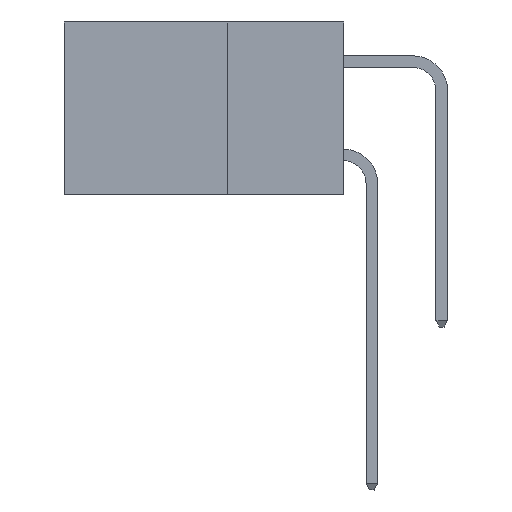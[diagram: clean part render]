
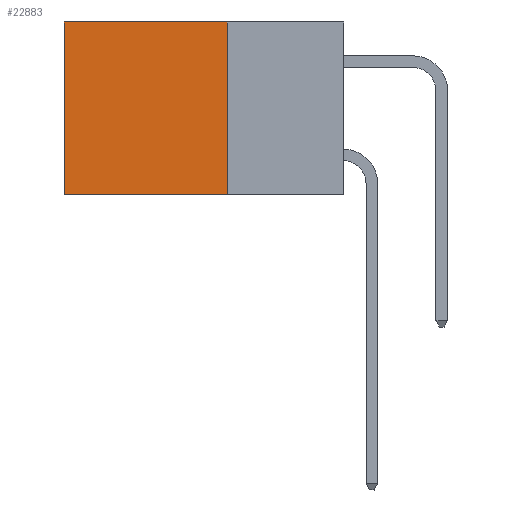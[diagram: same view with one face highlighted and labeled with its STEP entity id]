
A CAD part, left-side view. The second image highlights one B-rep face of the part: STEP entity #22883.
In plain terms, the highlighted planar face has unit normal (-1, 0, 0).
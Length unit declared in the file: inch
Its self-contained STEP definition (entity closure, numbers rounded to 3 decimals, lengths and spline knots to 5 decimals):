
#1088 = DIRECTION ( 'NONE',  ( 0., 0., -1. ) ) ;
#2029 = CARTESIAN_POINT ( 'NONE',  ( 0.298, 0.6, 0. ) ) ;
#2902 = VECTOR ( 'NONE', #4752, 39.37008 ) ;
#3681 = DIRECTION ( 'NONE',  ( 1., 0., 0. ) ) ;
#4088 = VECTOR ( 'NONE', #13898, 39.37008 ) ;
#4752 = DIRECTION ( 'NONE',  ( 0., 0., -1. ) ) ;
#5092 = DIRECTION ( 'NONE',  ( 0., 1., 0. ) ) ;
#6808 = VERTEX_POINT ( 'NONE', #8067 ) ;
#7173 = LINE ( 'NONE', #2029, #2902 ) ;
#8067 = CARTESIAN_POINT ( 'NONE',  ( 0.298, 0.6, -0.37 ) ) ;
#9467 = VECTOR ( 'NONE', #14996, 39.37008 ) ;
#9602 = CARTESIAN_POINT ( 'NONE',  ( 0.298, 0.25, 0. ) ) ;
#10108 = EDGE_CURVE ( 'NONE', #17441, #6808, #19126, .T. ) ;
#12580 = ORIENTED_EDGE ( 'NONE', *, *, #15314, .T. ) ;
#12760 = VECTOR ( 'NONE', #5092, 39.37008 ) ;
#12767 = CARTESIAN_POINT ( 'NONE',  ( 0.298, 0.6, 0. ) ) ;
#13898 = DIRECTION ( 'NONE',  ( 0., 1., 0. ) ) ;
#13939 = EDGE_LOOP ( 'NONE', ( #32686, #33712, #18588, #12580 ) ) ;
#14545 = CARTESIAN_POINT ( 'NONE',  ( 0.298, 0.25, 0. ) ) ;
#14996 = DIRECTION ( 'NONE',  ( 0., 0., -1. ) ) ;
#15314 = EDGE_CURVE ( 'NONE', #25634, #25080, #19343, .T. ) ;
#17277 = PLANE ( 'NONE',  #24728 ) ;
#17441 = VERTEX_POINT ( 'NONE', #31121 ) ;
#18588 = ORIENTED_EDGE ( 'NONE', *, *, #22995, .F. ) ;
#19126 = LINE ( 'NONE', #21307, #12760 ) ;
#19343 = LINE ( 'NONE', #30182, #4088 ) ;
#21307 = CARTESIAN_POINT ( 'NONE',  ( 0.298, 0.25, -0.37 ) ) ;
#22883 = ADVANCED_FACE ( 'NONE', ( #27292 ), #17277, .F. ) ;
#22995 = EDGE_CURVE ( 'NONE', #25634, #17441, #31943, .T. ) ;
#23186 = CARTESIAN_POINT ( 'NONE',  ( 0.298, 0.25, 0. ) ) ;
#24728 = AXIS2_PLACEMENT_3D ( 'NONE', #14545, #3681, #1088 ) ;
#25080 = VERTEX_POINT ( 'NONE', #12767 ) ;
#25088 = EDGE_CURVE ( 'NONE', #25080, #6808, #7173, .T. ) ;
#25634 = VERTEX_POINT ( 'NONE', #23186 ) ;
#27292 = FACE_OUTER_BOUND ( 'NONE', #13939, .T. ) ;
#30182 = CARTESIAN_POINT ( 'NONE',  ( 0.298, 0.25, 0. ) ) ;
#31121 = CARTESIAN_POINT ( 'NONE',  ( 0.298, 0.25, -0.37 ) ) ;
#31943 = LINE ( 'NONE', #9602, #9467 ) ;
#32686 = ORIENTED_EDGE ( 'NONE', *, *, #25088, .T. ) ;
#33712 = ORIENTED_EDGE ( 'NONE', *, *, #10108, .F. ) ;
